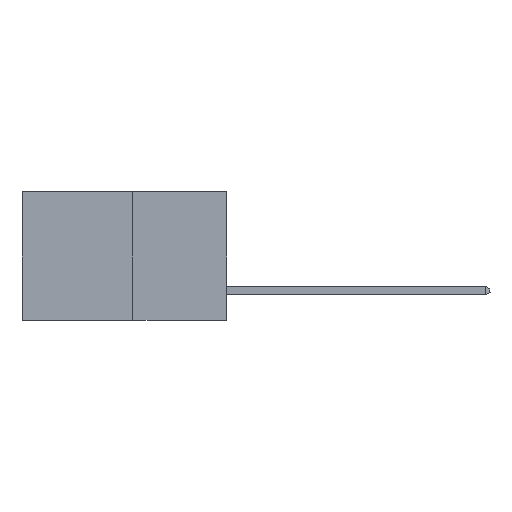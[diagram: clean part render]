
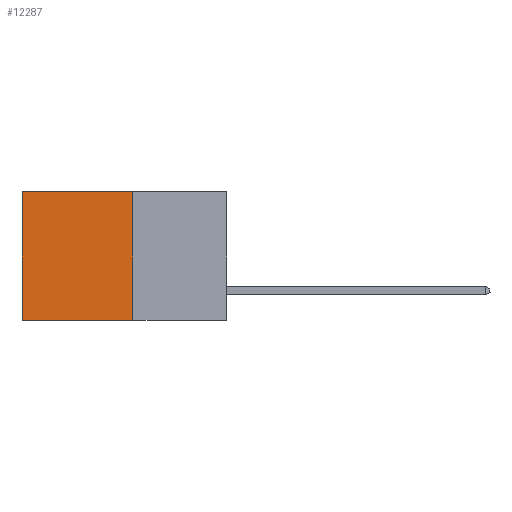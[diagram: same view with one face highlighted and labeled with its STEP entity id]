
A CAD part, left-side view. The second image highlights one B-rep face of the part: STEP entity #12287.
In plain terms, the highlighted planar face has unit normal (-1, 0, 0).
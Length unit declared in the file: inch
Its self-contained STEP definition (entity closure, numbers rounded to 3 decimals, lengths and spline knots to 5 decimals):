
#256 = VECTOR ( 'NONE', #2284, 39.37008 ) ;
#589 = DIRECTION ( 'NONE',  ( 0., 0., -1. ) ) ;
#639 = CARTESIAN_POINT ( 'NONE',  ( 0.277, 0.27, -0.37 ) ) ;
#798 = DIRECTION ( 'NONE',  ( 0., 0., -1. ) ) ;
#1144 = EDGE_LOOP ( 'NONE', ( #1187, #2088, #4319, #14296 ) ) ;
#1187 = ORIENTED_EDGE ( 'NONE', *, *, #12568, .T. ) ;
#2088 = ORIENTED_EDGE ( 'NONE', *, *, #11049, .F. ) ;
#2284 = DIRECTION ( 'NONE',  ( 0., 1., 0. ) ) ;
#2386 = CARTESIAN_POINT ( 'NONE',  ( 0.277, 0.27, -0.37 ) ) ;
#2848 = LINE ( 'NONE', #4645, #11473 ) ;
#2881 = VERTEX_POINT ( 'NONE', #12264 ) ;
#3305 = CARTESIAN_POINT ( 'NONE',  ( 0.277, 0.59, 0. ) ) ;
#3599 = DIRECTION ( 'NONE',  ( 0., 1., 0. ) ) ;
#3791 = FACE_OUTER_BOUND ( 'NONE', #1144, .T. ) ;
#4319 = ORIENTED_EDGE ( 'NONE', *, *, #13849, .F. ) ;
#4645 = CARTESIAN_POINT ( 'NONE',  ( 0.277, 0.59, -0.37 ) ) ;
#4984 = EDGE_CURVE ( 'NONE', #2881, #8412, #6141, .T. ) ;
#5654 = LINE ( 'NONE', #2386, #11209 ) ;
#5821 = DIRECTION ( 'NONE',  ( 0., 0., -1. ) ) ;
#6141 = LINE ( 'NONE', #6586, #256 ) ;
#6586 = CARTESIAN_POINT ( 'NONE',  ( 0.277, 0.27, 0. ) ) ;
#7573 = DIRECTION ( 'NONE',  ( 1., 0., 0. ) ) ;
#8412 = VERTEX_POINT ( 'NONE', #3305 ) ;
#8545 = AXIS2_PLACEMENT_3D ( 'NONE', #13853, #7573, #589 ) ;
#9520 = VERTEX_POINT ( 'NONE', #639 ) ;
#9754 = PLANE ( 'NONE',  #8545 ) ;
#9768 = VECTOR ( 'NONE', #798, 39.37008 ) ;
#11049 = EDGE_CURVE ( 'NONE', #9520, #11749, #5654, .T. ) ;
#11209 = VECTOR ( 'NONE', #3599, 39.37008 ) ;
#11473 = VECTOR ( 'NONE', #5821, 39.37008 ) ;
#11749 = VERTEX_POINT ( 'NONE', #13534 ) ;
#12264 = CARTESIAN_POINT ( 'NONE',  ( 0.277, 0.27, 0. ) ) ;
#12287 = ADVANCED_FACE ( 'NONE', ( #3791 ), #9754, .F. ) ;
#12568 = EDGE_CURVE ( 'NONE', #8412, #11749, #2848, .T. ) ;
#12796 = LINE ( 'NONE', #14030, #9768 ) ;
#13534 = CARTESIAN_POINT ( 'NONE',  ( 0.277, 0.59, -0.37 ) ) ;
#13849 = EDGE_CURVE ( 'NONE', #2881, #9520, #12796, .T. ) ;
#13853 = CARTESIAN_POINT ( 'NONE',  ( 0.277, 0.27, -0.37 ) ) ;
#14030 = CARTESIAN_POINT ( 'NONE',  ( 0.277, 0.27, -0.37 ) ) ;
#14296 = ORIENTED_EDGE ( 'NONE', *, *, #4984, .T. ) ;
